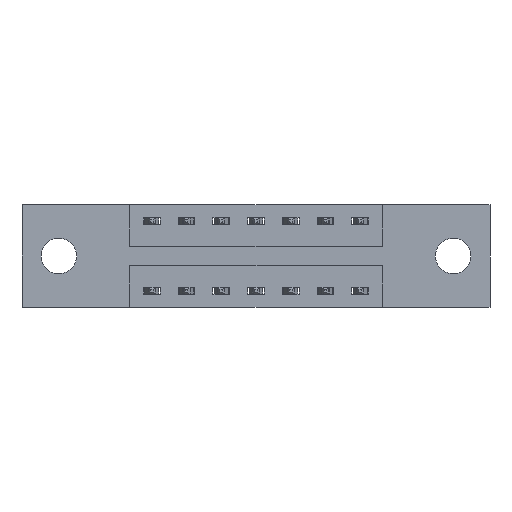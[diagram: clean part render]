
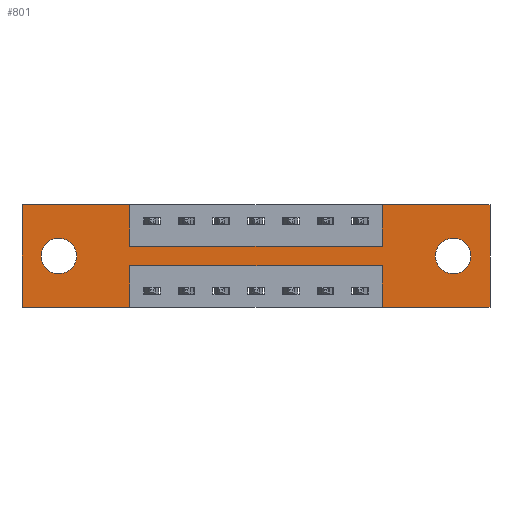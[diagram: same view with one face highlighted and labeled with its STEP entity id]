
A CAD part, front view. The second image highlights one B-rep face of the part: STEP entity #801.
In plain terms, the highlighted planar face has unit normal (0, -1, 0).
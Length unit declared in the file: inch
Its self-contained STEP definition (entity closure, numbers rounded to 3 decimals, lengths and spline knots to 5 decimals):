
#34 = CARTESIAN_POINT ( 'NONE',  ( 0.3875, 0., -0.22 ) ) ;
#56 = DIRECTION ( 'NONE',  ( 1., 0., 0. ) ) ;
#102 = VERTEX_POINT ( 'NONE', #4503 ) ;
#171 = EDGE_CURVE ( 'NONE', #5653, #6367, #6743, .T. ) ;
#192 = EDGE_CURVE ( 'NONE', #5368, #5728, #2642, .T. ) ;
#245 = VERTEX_POINT ( 'NONE', #8207 ) ;
#246 = EDGE_CURVE ( 'NONE', #5728, #825, #8740, .T. ) ;
#260 = EDGE_CURVE ( 'NONE', #6367, #8757, #5092, .T. ) ;
#282 = EDGE_CURVE ( 'NONE', #3865, #5653, #7958, .T. ) ;
#293 = CARTESIAN_POINT ( 'NONE',  ( 0.3875, 0., -0.15 ) ) ;
#325 = EDGE_CURVE ( 'NONE', #649, #1746, #8823, .T. ) ;
#329 = CARTESIAN_POINT ( 'NONE',  ( 0.3875, 0., -0.37 ) ) ;
#339 = EDGE_CURVE ( 'NONE', #2896, #6862, #3319, .T. ) ;
#341 = EDGE_CURVE ( 'NONE', #102, #3865, #3550, .T. ) ;
#356 = EDGE_CURVE ( 'NONE', #2220, #102, #3084, .T. ) ;
#359 = EDGE_CURVE ( 'NONE', #825, #2220, #8264, .T. ) ;
#379 = EDGE_CURVE ( 'NONE', #4801, #5236, #4547, .T. ) ;
#402 = EDGE_CURVE ( 'NONE', #245, #4801, #8917, .T. ) ;
#419 = EDGE_CURVE ( 'NONE', #8757, #245, #7037, .T. ) ;
#572 = DIRECTION ( 'NONE',  ( 0., 0., 1. ) ) ;
#649 = VERTEX_POINT ( 'NONE', #4468 ) ;
#759 = DIRECTION ( 'NONE',  ( 0., 0., -1. ) ) ;
#801 = ADVANCED_FACE ( 'NONE', ( #8259, #6731, #2843 ), #5018, .T. ) ;
#825 = VERTEX_POINT ( 'NONE', #3367 ) ;
#1147 = AXIS2_PLACEMENT_3D ( 'NONE', #3128, #7862, #3862 ) ;
#1239 = CARTESIAN_POINT ( 'NONE',  ( 1.685, 0., 0. ) ) ;
#1423 = AXIS2_PLACEMENT_3D ( 'NONE', #3573, #8265, #4294 ) ;
#1541 = CARTESIAN_POINT ( 'NONE',  ( 1.2975, 0., -0.22 ) ) ;
#1558 = EDGE_CURVE ( 'NONE', #5236, #5368, #9074, .T. ) ;
#1677 = EDGE_LOOP ( 'NONE', ( #3894, #3574, #3557, #4781, #4130, #3641, #3634, #3622, #3614, #3603, #6027, #5846 ) ) ;
#1746 = VERTEX_POINT ( 'NONE', #4583 ) ;
#1949 = CARTESIAN_POINT ( 'NONE',  ( 0.1325, 0., -0.249 ) ) ;
#1970 = DIRECTION ( 'NONE',  ( 0., 0., 1. ) ) ;
#2023 = AXIS2_PLACEMENT_3D ( 'NONE', #4751, #6834, #7574 ) ;
#2156 = ORIENTED_EDGE ( 'NONE', *, *, #325, .T. ) ;
#2187 = ORIENTED_EDGE ( 'NONE', *, *, #6342, .T. ) ;
#2220 = VERTEX_POINT ( 'NONE', #1541 ) ;
#2634 = VECTOR ( 'NONE', #3242, 39.37008 ) ;
#2642 = LINE ( 'NONE', #1239, #6146 ) ;
#2643 = DIRECTION ( 'NONE',  ( 0., 0., -1. ) ) ;
#2836 = DIRECTION ( 'NONE',  ( 0., -1., 0. ) ) ;
#2843 = FACE_OUTER_BOUND ( 'NONE', #1677, .T. ) ;
#2849 = VECTOR ( 'NONE', #1970, 39.37008 ) ;
#2896 = VERTEX_POINT ( 'NONE', #3766 ) ;
#2978 = CARTESIAN_POINT ( 'NONE',  ( 0.1325, 0., -0.185 ) ) ;
#3047 = CARTESIAN_POINT ( 'NONE',  ( 1.2975, 0., 0. ) ) ;
#3064 = CIRCLE ( 'NONE', #1147, 0.064 ) ;
#3080 = CIRCLE ( 'NONE', #1423, 0.064 ) ;
#3084 = LINE ( 'NONE', #34, #4985 ) ;
#3128 = CARTESIAN_POINT ( 'NONE',  ( 1.5525, 0., -0.185 ) ) ;
#3170 = CARTESIAN_POINT ( 'NONE',  ( 0., 0., 0. ) ) ;
#3208 = VECTOR ( 'NONE', #56, 39.37008 ) ;
#3242 = DIRECTION ( 'NONE',  ( 0., 0., 1. ) ) ;
#3319 = CIRCLE ( 'NONE', #3886, 0.064 ) ;
#3367 = CARTESIAN_POINT ( 'NONE',  ( 1.2975, 0., -0.37 ) ) ;
#3420 = CARTESIAN_POINT ( 'NONE',  ( 0.3875, 0., -0.37 ) ) ;
#3550 = LINE ( 'NONE', #3420, #6738 ) ;
#3557 = ORIENTED_EDGE ( 'NONE', *, *, #359, .F. ) ;
#3573 = CARTESIAN_POINT ( 'NONE',  ( 0.1325, 0., -0.185 ) ) ;
#3574 = ORIENTED_EDGE ( 'NONE', *, *, #356, .F. ) ;
#3603 = ORIENTED_EDGE ( 'NONE', *, *, #260, .F. ) ;
#3614 = ORIENTED_EDGE ( 'NONE', *, *, #419, .F. ) ;
#3622 = ORIENTED_EDGE ( 'NONE', *, *, #402, .F. ) ;
#3623 = CARTESIAN_POINT ( 'NONE',  ( 0., 0., 0. ) ) ;
#3634 = ORIENTED_EDGE ( 'NONE', *, *, #379, .F. ) ;
#3641 = ORIENTED_EDGE ( 'NONE', *, *, #1558, .F. ) ;
#3766 = CARTESIAN_POINT ( 'NONE',  ( 0.1325, 0., -0.121 ) ) ;
#3794 = DIRECTION ( 'NONE',  ( -1., 0., 0. ) ) ;
#3828 = CARTESIAN_POINT ( 'NONE',  ( 1.2975, 0., -0.37 ) ) ;
#3862 = DIRECTION ( 'NONE',  ( 0., 0., -1. ) ) ;
#3865 = VERTEX_POINT ( 'NONE', #329 ) ;
#3879 = VECTOR ( 'NONE', #7890, 39.37008 ) ;
#3886 = AXIS2_PLACEMENT_3D ( 'NONE', #2978, #8824, #7052 ) ;
#3894 = ORIENTED_EDGE ( 'NONE', *, *, #341, .F. ) ;
#3902 = ORIENTED_EDGE ( 'NONE', *, *, #4473, .T. ) ;
#4096 = ORIENTED_EDGE ( 'NONE', *, *, #339, .T. ) ;
#4130 = ORIENTED_EDGE ( 'NONE', *, *, #192, .F. ) ;
#4294 = DIRECTION ( 'NONE',  ( 0., 0., 1. ) ) ;
#4441 = VECTOR ( 'NONE', #3794, 39.37008 ) ;
#4468 = CARTESIAN_POINT ( 'NONE',  ( 1.5525, 0., -0.121 ) ) ;
#4473 = EDGE_CURVE ( 'NONE', #6862, #2896, #3080, .T. ) ;
#4503 = CARTESIAN_POINT ( 'NONE',  ( 0.3875, 0., -0.22 ) ) ;
#4547 = LINE ( 'NONE', #3047, #2634 ) ;
#4583 = CARTESIAN_POINT ( 'NONE',  ( 1.5525, 0., -0.249 ) ) ;
#4613 = CARTESIAN_POINT ( 'NONE',  ( 0., 0., -0.37 ) ) ;
#4653 = CARTESIAN_POINT ( 'NONE',  ( 0.3875, 0., 0. ) ) ;
#4751 = CARTESIAN_POINT ( 'NONE',  ( 1.5525, 0., -0.185 ) ) ;
#4781 = ORIENTED_EDGE ( 'NONE', *, *, #246, .F. ) ;
#4801 = VERTEX_POINT ( 'NONE', #5323 ) ;
#4985 = VECTOR ( 'NONE', #7313, 39.37008 ) ;
#5018 = PLANE ( 'NONE',  #7310 ) ;
#5092 = LINE ( 'NONE', #3170, #3208 ) ;
#5157 = CARTESIAN_POINT ( 'NONE',  ( 1.685, 0., 0. ) ) ;
#5236 = VERTEX_POINT ( 'NONE', #6998 ) ;
#5323 = CARTESIAN_POINT ( 'NONE',  ( 1.2975, 0., -0.15 ) ) ;
#5368 = VERTEX_POINT ( 'NONE', #5157 ) ;
#5411 = CARTESIAN_POINT ( 'NONE',  ( 1.685, 0., -0.37 ) ) ;
#5564 = EDGE_LOOP ( 'NONE', ( #2156, #2187 ) ) ;
#5608 = CARTESIAN_POINT ( 'NONE',  ( 0.3875, 0., 0. ) ) ;
#5653 = VERTEX_POINT ( 'NONE', #9198 ) ;
#5707 = CARTESIAN_POINT ( 'NONE',  ( 0., 0., 0. ) ) ;
#5728 = VERTEX_POINT ( 'NONE', #5411 ) ;
#5846 = ORIENTED_EDGE ( 'NONE', *, *, #282, .F. ) ;
#5866 = DIRECTION ( 'NONE',  ( 0., 0., -1. ) ) ;
#6027 = ORIENTED_EDGE ( 'NONE', *, *, #171, .F. ) ;
#6146 = VECTOR ( 'NONE', #759, 39.37008 ) ;
#6342 = EDGE_CURVE ( 'NONE', #1746, #649, #3064, .T. ) ;
#6367 = VERTEX_POINT ( 'NONE', #8501 ) ;
#6731 = FACE_BOUND ( 'NONE', #9192, .T. ) ;
#6738 = VECTOR ( 'NONE', #2643, 39.37008 ) ;
#6743 = LINE ( 'NONE', #3623, #8270 ) ;
#6834 = DIRECTION ( 'NONE',  ( 0., 1., 0. ) ) ;
#6862 = VERTEX_POINT ( 'NONE', #1949 ) ;
#6977 = DIRECTION ( 'NONE',  ( 0., 0., -1. ) ) ;
#6998 = CARTESIAN_POINT ( 'NONE',  ( 1.2975, 0., 0. ) ) ;
#7037 = LINE ( 'NONE', #5608, #8733 ) ;
#7052 = DIRECTION ( 'NONE',  ( 0., 0., 1. ) ) ;
#7196 = VECTOR ( 'NONE', #8285, 39.37008 ) ;
#7310 = AXIS2_PLACEMENT_3D ( 'NONE', #8648, #2836, #6977 ) ;
#7313 = DIRECTION ( 'NONE',  ( -1., 0., 0. ) ) ;
#7574 = DIRECTION ( 'NONE',  ( 0., 0., -1. ) ) ;
#7698 = CARTESIAN_POINT ( 'NONE',  ( 0., 0., -0.37 ) ) ;
#7862 = DIRECTION ( 'NONE',  ( 0., 1., 0. ) ) ;
#7890 = DIRECTION ( 'NONE',  ( 1., 0., 0. ) ) ;
#7958 = LINE ( 'NONE', #4613, #4441 ) ;
#8207 = CARTESIAN_POINT ( 'NONE',  ( 0.3875, 0., -0.15 ) ) ;
#8259 = FACE_BOUND ( 'NONE', #5564, .T. ) ;
#8264 = LINE ( 'NONE', #3828, #2849 ) ;
#8265 = DIRECTION ( 'NONE',  ( 0., 1., 0. ) ) ;
#8270 = VECTOR ( 'NONE', #572, 39.37008 ) ;
#8285 = DIRECTION ( 'NONE',  ( 1., 0., 0. ) ) ;
#8501 = CARTESIAN_POINT ( 'NONE',  ( 0., 0., 0. ) ) ;
#8556 = VECTOR ( 'NONE', #9096, 39.37008 ) ;
#8648 = CARTESIAN_POINT ( 'NONE',  ( 0., 0., -0.37 ) ) ;
#8733 = VECTOR ( 'NONE', #5866, 39.37008 ) ;
#8740 = LINE ( 'NONE', #7698, #8556 ) ;
#8757 = VERTEX_POINT ( 'NONE', #4653 ) ;
#8823 = CIRCLE ( 'NONE', #2023, 0.064 ) ;
#8824 = DIRECTION ( 'NONE',  ( 0., 1., 0. ) ) ;
#8917 = LINE ( 'NONE', #293, #3879 ) ;
#9074 = LINE ( 'NONE', #5707, #7196 ) ;
#9096 = DIRECTION ( 'NONE',  ( -1., 0., 0. ) ) ;
#9192 = EDGE_LOOP ( 'NONE', ( #4096, #3902 ) ) ;
#9198 = CARTESIAN_POINT ( 'NONE',  ( 0., 0., -0.37 ) ) ;
